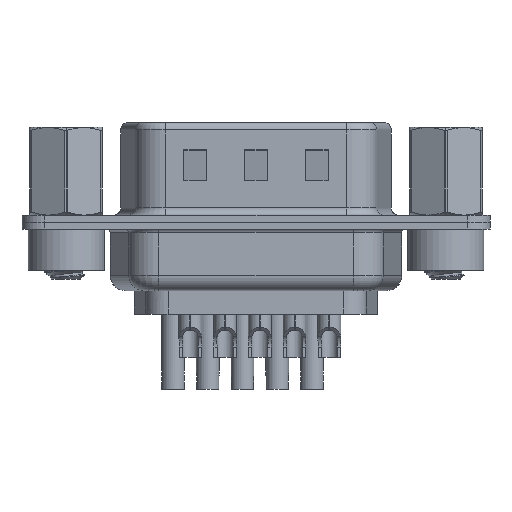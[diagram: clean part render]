
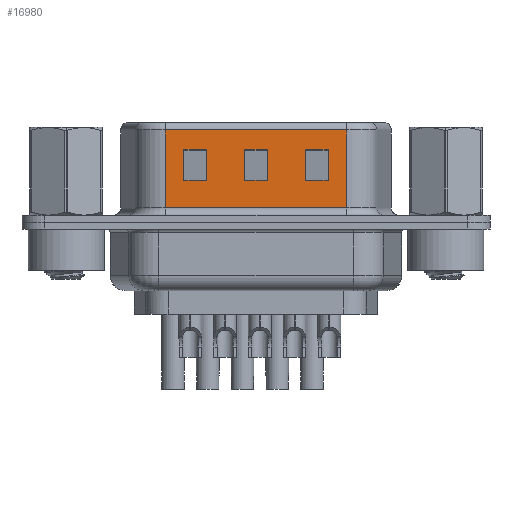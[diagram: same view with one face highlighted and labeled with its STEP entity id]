
A CAD part, front view. The second image highlights one B-rep face of the part: STEP entity #16980.
In plain terms, the highlighted planar face has unit normal (0, -1, 0).
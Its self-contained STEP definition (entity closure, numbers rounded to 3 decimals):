
#253 = DIRECTION ( 'NONE',  ( 0., 0., -1. ) ) ;
#734 = VERTEX_POINT ( 'NONE', #9181 ) ;
#1091 = FACE_BOUND ( 'NONE', #15045, .T. ) ;
#1132 = DIRECTION ( 'NONE',  ( 1., 0., 0. ) ) ;
#1207 = FACE_BOUND ( 'NONE', #1590, .T. ) ;
#1249 = ORIENTED_EDGE ( 'NONE', *, *, #4398, .T. ) ;
#1345 = EDGE_CURVE ( 'NONE', #5657, #16058, #13786, .T. ) ;
#1434 = VECTOR ( 'NONE', #18201, 1000. ) ;
#1453 = DIRECTION ( 'NONE',  ( 0., 1., 0. ) ) ;
#1513 = VECTOR ( 'NONE', #1132, 1000. ) ;
#1590 = EDGE_LOOP ( 'NONE', ( #18565, #24403, #11874, #5503 ) ) ;
#2012 = ORIENTED_EDGE ( 'NONE', *, *, #1345, .T. ) ;
#2089 = VERTEX_POINT ( 'NONE', #5091 ) ;
#2094 = EDGE_CURVE ( 'NONE', #13016, #23794, #4855, .T. ) ;
#2251 = CARTESIAN_POINT ( 'NONE',  ( 13.245, -4.64, 6.57 ) ) ;
#2502 = DIRECTION ( 'NONE',  ( 0., 0., -1. ) ) ;
#3294 = ORIENTED_EDGE ( 'NONE', *, *, #21431, .T. ) ;
#3362 = VERTEX_POINT ( 'NONE', #21740 ) ;
#3527 = LINE ( 'NONE', #14762, #15065 ) ;
#3961 = LINE ( 'NONE', #22875, #13768 ) ;
#3984 = DIRECTION ( 'NONE',  ( 0., 0., -1. ) ) ;
#4079 = CARTESIAN_POINT ( 'NONE',  ( 22.474, -4.64, 2.755 ) ) ;
#4138 = VERTEX_POINT ( 'NONE', #21803 ) ;
#4312 = VECTOR ( 'NONE', #8148, 1000. ) ;
#4398 = EDGE_CURVE ( 'NONE', #22887, #10672, #21528, .T. ) ;
#4487 = LINE ( 'NONE', #19798, #13297 ) ;
#4555 = DIRECTION ( 'NONE',  ( 0., 0., -1. ) ) ;
#4747 = CARTESIAN_POINT ( 'NONE',  ( 11.745, -4.64, 4.755 ) ) ;
#4855 = LINE ( 'NONE', #8548, #21763 ) ;
#4895 = CARTESIAN_POINT ( 'NONE',  ( 18.474, -4.64, 6.07 ) ) ;
#5091 = CARTESIAN_POINT ( 'NONE',  ( 9.245, -4.64, 2.755 ) ) ;
#5443 = AXIS2_PLACEMENT_3D ( 'NONE', #11084, #1453, #24064 ) ;
#5503 = ORIENTED_EDGE ( 'NONE', *, *, #2094, .T. ) ;
#5657 = VERTEX_POINT ( 'NONE', #23754 ) ;
#5834 = LINE ( 'NONE', #2251, #6319 ) ;
#6092 = DIRECTION ( 'NONE',  ( 1., 0., 0. ) ) ;
#6319 = VECTOR ( 'NONE', #3984, 1000. ) ;
#6425 = VERTEX_POINT ( 'NONE', #18250 ) ;
#6822 = DIRECTION ( 'NONE',  ( 1., 0., 0. ) ) ;
#6982 = DIRECTION ( 'NONE',  ( -1., 0., 0. ) ) ;
#7063 = VERTEX_POINT ( 'NONE', #13163 ) ;
#8148 = DIRECTION ( 'NONE',  ( -1., 0., 0. ) ) ;
#8548 = CARTESIAN_POINT ( 'NONE',  ( 11.745, -4.64, 6.57 ) ) ;
#8857 = PLANE ( 'NONE',  #5443 ) ;
#9181 = CARTESIAN_POINT ( 'NONE',  ( 6.516, -4.64, 0.95 ) ) ;
#9366 = CARTESIAN_POINT ( 'NONE',  ( 11.745, -4.64, 2.755 ) ) ;
#9613 = EDGE_CURVE ( 'NONE', #16058, #22887, #22147, .T. ) ;
#9751 = LINE ( 'NONE', #4079, #4312 ) ;
#9788 = LINE ( 'NONE', #23028, #21166 ) ;
#10103 = ORIENTED_EDGE ( 'NONE', *, *, #12237, .T. ) ;
#10149 = CARTESIAN_POINT ( 'NONE',  ( 17.245, -4.64, 6.57 ) ) ;
#10470 = VECTOR ( 'NONE', #24336, 1000. ) ;
#10630 = CARTESIAN_POINT ( 'NONE',  ( 14.474, -4.64, 4.755 ) ) ;
#10672 = VERTEX_POINT ( 'NONE', #15716 ) ;
#10965 = CARTESIAN_POINT ( 'NONE',  ( 17.245, -4.64, 4.755 ) ) ;
#10969 = EDGE_LOOP ( 'NONE', ( #11867, #11568, #3294, #21873 ) ) ;
#11048 = CARTESIAN_POINT ( 'NONE',  ( 7.745, -4.64, 6.57 ) ) ;
#11084 = CARTESIAN_POINT ( 'NONE',  ( 18.474, -4.64, 6.57 ) ) ;
#11568 = ORIENTED_EDGE ( 'NONE', *, *, #11924, .T. ) ;
#11637 = VERTEX_POINT ( 'NONE', #4895 ) ;
#11810 = EDGE_CURVE ( 'NONE', #10672, #5657, #9751, .T. ) ;
#11867 = ORIENTED_EDGE ( 'NONE', *, *, #18592, .F. ) ;
#11874 = ORIENTED_EDGE ( 'NONE', *, *, #14469, .T. ) ;
#11924 = EDGE_CURVE ( 'NONE', #11637, #17825, #13021, .T. ) ;
#11965 = LINE ( 'NONE', #23337, #20533 ) ;
#12237 = EDGE_CURVE ( 'NONE', #20249, #3362, #23865, .T. ) ;
#12642 = LINE ( 'NONE', #19819, #1434 ) ;
#12652 = VERTEX_POINT ( 'NONE', #21367 ) ;
#13016 = VERTEX_POINT ( 'NONE', #9366 ) ;
#13021 = LINE ( 'NONE', #13135, #14543 ) ;
#13135 = CARTESIAN_POINT ( 'NONE',  ( 18.474, -4.64, 6.07 ) ) ;
#13163 = CARTESIAN_POINT ( 'NONE',  ( 18.474, -4.64, 0.95 ) ) ;
#13297 = VECTOR ( 'NONE', #21536, 1000. ) ;
#13768 = VECTOR ( 'NONE', #253, 1000. ) ;
#13786 = LINE ( 'NONE', #15641, #20151 ) ;
#14469 = EDGE_CURVE ( 'NONE', #12652, #13016, #18641, .T. ) ;
#14543 = VECTOR ( 'NONE', #20919, 1000. ) ;
#14762 = CARTESIAN_POINT ( 'NONE',  ( 14.474, -4.64, 2.755 ) ) ;
#15045 = EDGE_LOOP ( 'NONE', ( #1249, #16280, #2012, #18392 ) ) ;
#15058 = EDGE_CURVE ( 'NONE', #23794, #6425, #12642, .T. ) ;
#15065 = VECTOR ( 'NONE', #6982, 1000. ) ;
#15246 = VECTOR ( 'NONE', #18581, 1000. ) ;
#15258 = EDGE_CURVE ( 'NONE', #4138, #20249, #16460, .T. ) ;
#15459 = EDGE_CURVE ( 'NONE', #734, #7063, #9788, .T. ) ;
#15556 = ORIENTED_EDGE ( 'NONE', *, *, #15258, .T. ) ;
#15641 = CARTESIAN_POINT ( 'NONE',  ( 15.745, -4.64, 6.57 ) ) ;
#15716 = CARTESIAN_POINT ( 'NONE',  ( 17.245, -4.64, 2.755 ) ) ;
#15981 = EDGE_CURVE ( 'NONE', #3362, #2089, #4487, .T. ) ;
#16058 = VERTEX_POINT ( 'NONE', #24375 ) ;
#16193 = CARTESIAN_POINT ( 'NONE',  ( 22.474, -4.64, 4.755 ) ) ;
#16280 = ORIENTED_EDGE ( 'NONE', *, *, #11810, .T. ) ;
#16419 = VECTOR ( 'NONE', #6822, 1000. ) ;
#16460 = LINE ( 'NONE', #11048, #15246 ) ;
#16536 = EDGE_LOOP ( 'NONE', ( #22344, #17729, #15556, #10103 ) ) ;
#16980 = ADVANCED_FACE ( 'NONE', ( #24191, #1091, #1207, #22347 ), #8857, .F. ) ;
#17438 = CARTESIAN_POINT ( 'NONE',  ( 7.745, -4.64, 4.755 ) ) ;
#17729 = ORIENTED_EDGE ( 'NONE', *, *, #23402, .T. ) ;
#17825 = VERTEX_POINT ( 'NONE', #19833 ) ;
#18051 = DIRECTION ( 'NONE',  ( 0., 0., 1. ) ) ;
#18201 = DIRECTION ( 'NONE',  ( 1., 0., 0. ) ) ;
#18250 = CARTESIAN_POINT ( 'NONE',  ( 13.245, -4.64, 4.755 ) ) ;
#18392 = ORIENTED_EDGE ( 'NONE', *, *, #9613, .T. ) ;
#18565 = ORIENTED_EDGE ( 'NONE', *, *, #15058, .T. ) ;
#18581 = DIRECTION ( 'NONE',  ( 0., 0., 1. ) ) ;
#18592 = EDGE_CURVE ( 'NONE', #11637, #7063, #3961, .T. ) ;
#18641 = LINE ( 'NONE', #18764, #10470 ) ;
#18764 = CARTESIAN_POINT ( 'NONE',  ( 18.474, -4.64, 2.755 ) ) ;
#19246 = DIRECTION ( 'NONE',  ( 0., 0., 1. ) ) ;
#19798 = CARTESIAN_POINT ( 'NONE',  ( 9.245, -4.64, 6.57 ) ) ;
#19819 = CARTESIAN_POINT ( 'NONE',  ( 18.474, -4.64, 4.755 ) ) ;
#19833 = CARTESIAN_POINT ( 'NONE',  ( 6.516, -4.64, 6.07 ) ) ;
#20151 = VECTOR ( 'NONE', #19246, 1000. ) ;
#20249 = VERTEX_POINT ( 'NONE', #17438 ) ;
#20533 = VECTOR ( 'NONE', #4555, 1000. ) ;
#20721 = EDGE_CURVE ( 'NONE', #6425, #12652, #5834, .T. ) ;
#20919 = DIRECTION ( 'NONE',  ( -1., 0., 0. ) ) ;
#21166 = VECTOR ( 'NONE', #6092, 1000. ) ;
#21367 = CARTESIAN_POINT ( 'NONE',  ( 13.245, -4.64, 2.755 ) ) ;
#21431 = EDGE_CURVE ( 'NONE', #17825, #734, #11965, .T. ) ;
#21528 = LINE ( 'NONE', #10149, #23040 ) ;
#21536 = DIRECTION ( 'NONE',  ( 0., 0., -1. ) ) ;
#21740 = CARTESIAN_POINT ( 'NONE',  ( 9.245, -4.64, 4.755 ) ) ;
#21763 = VECTOR ( 'NONE', #18051, 1000. ) ;
#21803 = CARTESIAN_POINT ( 'NONE',  ( 7.745, -4.64, 2.755 ) ) ;
#21873 = ORIENTED_EDGE ( 'NONE', *, *, #15459, .T. ) ;
#22147 = LINE ( 'NONE', #16193, #16419 ) ;
#22344 = ORIENTED_EDGE ( 'NONE', *, *, #15981, .T. ) ;
#22347 = FACE_OUTER_BOUND ( 'NONE', #10969, .T. ) ;
#22875 = CARTESIAN_POINT ( 'NONE',  ( 18.474, -4.64, 6.57 ) ) ;
#22887 = VERTEX_POINT ( 'NONE', #10965 ) ;
#23028 = CARTESIAN_POINT ( 'NONE',  ( 18.474, -4.64, 0.95 ) ) ;
#23040 = VECTOR ( 'NONE', #2502, 1000. ) ;
#23337 = CARTESIAN_POINT ( 'NONE',  ( 6.516, -4.64, 6.57 ) ) ;
#23402 = EDGE_CURVE ( 'NONE', #2089, #4138, #3527, .T. ) ;
#23754 = CARTESIAN_POINT ( 'NONE',  ( 15.745, -4.64, 2.755 ) ) ;
#23794 = VERTEX_POINT ( 'NONE', #4747 ) ;
#23865 = LINE ( 'NONE', #10630, #1513 ) ;
#24064 = DIRECTION ( 'NONE',  ( 0., 0., 1. ) ) ;
#24191 = FACE_BOUND ( 'NONE', #16536, .T. ) ;
#24336 = DIRECTION ( 'NONE',  ( -1., 0., 0. ) ) ;
#24375 = CARTESIAN_POINT ( 'NONE',  ( 15.745, -4.64, 4.755 ) ) ;
#24403 = ORIENTED_EDGE ( 'NONE', *, *, #20721, .T. ) ;
